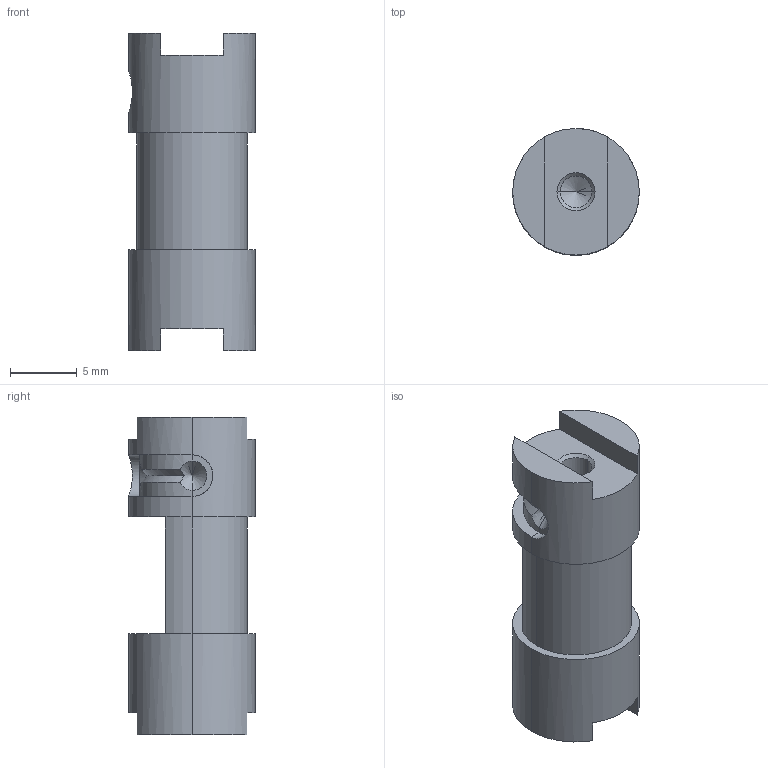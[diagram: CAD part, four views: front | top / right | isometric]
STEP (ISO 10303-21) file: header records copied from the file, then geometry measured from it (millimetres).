
FILE_DESCRIPTION (( 'STEP AP214' ), '1' );
FILE_NAME ('Selector.step', '2015-07-11T17:33:27', ( 'WarFairy' ), ( '' ), 'SwSTEP 2.0', 'SolidWorks 2015', '' );
FILE_SCHEMA (( 'AUTOMOTIVE_DESIGN' ));
Length unit declared in the file: millimetre
Products named in the file (1): Selector
Bounding box: 9.46 x 9.46 x 23.71 mm (x, y, z)
Volume: 1203.9 mm3; surface area: 982.5 mm2
Topology: 1 solids, 1 shells, 47 faces, 117 edges, 68 vertices
Faces by surface type: plane 17, cylinder 16, cone 14
Entity records: 1482 total; most frequent: CARTESIAN_POINT 314, DIRECTION 240, ORIENTED_EDGE 218, EDGE_CURVE 109, AXIS2_PLACEMENT_3D 94, VERTEX_POINT 68, VECTOR 52, LINE 52
